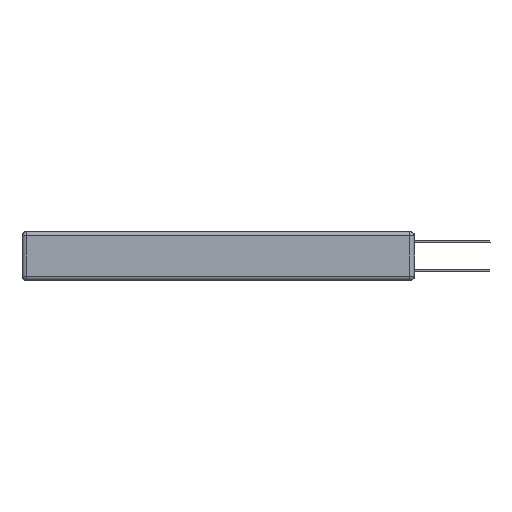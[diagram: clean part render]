
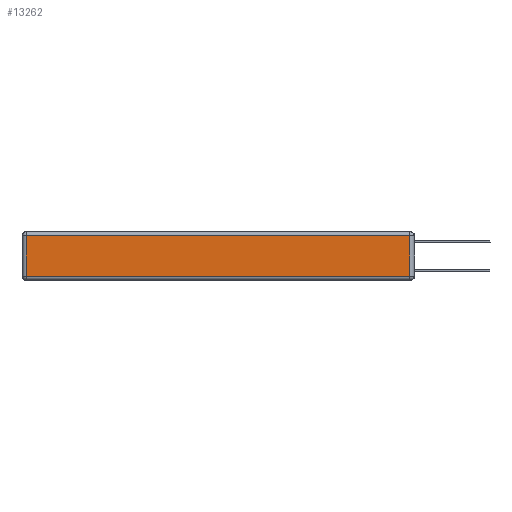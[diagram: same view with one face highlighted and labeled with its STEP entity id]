
A CAD part, left-side view. The second image highlights one B-rep face of the part: STEP entity #13262.
In plain terms, the highlighted planar face has unit normal (-1, 0, 0).
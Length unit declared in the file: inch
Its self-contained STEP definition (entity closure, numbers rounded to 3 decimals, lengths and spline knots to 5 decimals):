
#1195 = EDGE_CURVE ( 'NONE', #13569, #7701, #15950, .T. ) ;
#3044 = ORIENTED_EDGE ( 'NONE', *, *, #15689, .T. ) ;
#3171 = CARTESIAN_POINT ( 'NONE',  ( 0., 2.72, -0.03 ) ) ;
#3591 = EDGE_LOOP ( 'NONE', ( #12840, #3044, #17612, #6719 ) ) ;
#5031 = CARTESIAN_POINT ( 'NONE',  ( 0., 2.72, -0.313 ) ) ;
#5205 = PLANE ( 'NONE',  #25912 ) ;
#5471 = LINE ( 'NONE', #9842, #20085 ) ;
#6719 = ORIENTED_EDGE ( 'NONE', *, *, #12060, .T. ) ;
#6897 = DIRECTION ( 'NONE',  ( 0., 0., 1. ) ) ;
#7042 = CARTESIAN_POINT ( 'NONE',  ( 0., 0., -0.343 ) ) ;
#7701 = VERTEX_POINT ( 'NONE', #3171 ) ;
#7793 = VECTOR ( 'NONE', #25810, 39.37008 ) ;
#9604 = DIRECTION ( 'NONE',  ( 0., 1., 0. ) ) ;
#9842 = CARTESIAN_POINT ( 'NONE',  ( 0., 2.72, -0.343 ) ) ;
#10989 = VERTEX_POINT ( 'NONE', #16826 ) ;
#12060 = EDGE_CURVE ( 'NONE', #7701, #23189, #5471, .T. ) ;
#12840 = ORIENTED_EDGE ( 'NONE', *, *, #12869, .T. ) ;
#12869 = EDGE_CURVE ( 'NONE', #23189, #10989, #17781, .T. ) ;
#13262 = ADVANCED_FACE ( 'NONE', ( #22222 ), #5205, .T. ) ;
#13569 = VERTEX_POINT ( 'NONE', #15168 ) ;
#13958 = DIRECTION ( 'NONE',  ( 0., -1., 0. ) ) ;
#15168 = CARTESIAN_POINT ( 'NONE',  ( 0., 0.03, -0.03 ) ) ;
#15689 = EDGE_CURVE ( 'NONE', #10989, #13569, #25677, .T. ) ;
#15950 = LINE ( 'NONE', #22832, #23268 ) ;
#16454 = DIRECTION ( 'NONE',  ( 0., 0., -1. ) ) ;
#16826 = CARTESIAN_POINT ( 'NONE',  ( 0., 0.03, -0.313 ) ) ;
#17612 = ORIENTED_EDGE ( 'NONE', *, *, #1195, .T. ) ;
#17744 = DIRECTION ( 'NONE',  ( -1., 0., 0. ) ) ;
#17781 = LINE ( 'NONE', #22258, #21904 ) ;
#20085 = VECTOR ( 'NONE', #16454, 39.37008 ) ;
#21904 = VECTOR ( 'NONE', #13958, 39.37008 ) ;
#22222 = FACE_OUTER_BOUND ( 'NONE', #3591, .T. ) ;
#22258 = CARTESIAN_POINT ( 'NONE',  ( 0., 0., -0.313 ) ) ;
#22832 = CARTESIAN_POINT ( 'NONE',  ( 0., 2.75, -0.03 ) ) ;
#23137 = CARTESIAN_POINT ( 'NONE',  ( 0., 0.03, -0.343 ) ) ;
#23189 = VERTEX_POINT ( 'NONE', #5031 ) ;
#23268 = VECTOR ( 'NONE', #9604, 39.37008 ) ;
#25677 = LINE ( 'NONE', #23137, #7793 ) ;
#25810 = DIRECTION ( 'NONE',  ( 0., 0., 1. ) ) ;
#25912 = AXIS2_PLACEMENT_3D ( 'NONE', #7042, #17744, #6897 ) ;
